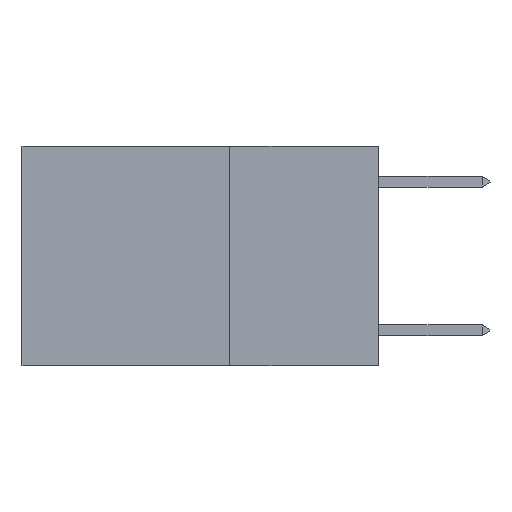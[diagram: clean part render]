
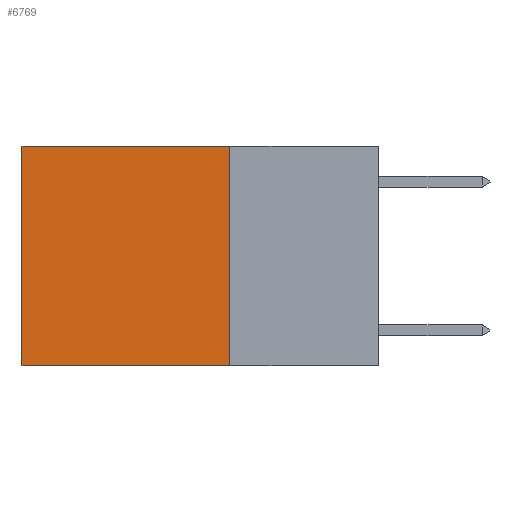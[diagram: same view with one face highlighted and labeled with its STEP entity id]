
A CAD part, left-side view. The second image highlights one B-rep face of the part: STEP entity #6769.
In plain terms, the highlighted planar face has unit normal (-1, 0, 0).
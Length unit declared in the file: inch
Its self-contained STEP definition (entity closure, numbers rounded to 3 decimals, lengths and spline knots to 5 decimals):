
#314 = CARTESIAN_POINT ( 'NONE',  ( 0.2625, 0.6, 0. ) ) ;
#1008 = DIRECTION ( 'NONE',  ( 1., 0., 0. ) ) ;
#1084 = LINE ( 'NONE', #8277, #3720 ) ;
#1279 = VERTEX_POINT ( 'NONE', #1450 ) ;
#1300 = ORIENTED_EDGE ( 'NONE', *, *, #3830, .T. ) ;
#1450 = CARTESIAN_POINT ( 'NONE',  ( 0.2625, 0.6, -0.37 ) ) ;
#1474 = DIRECTION ( 'NONE',  ( 0., 0., -1. ) ) ;
#1556 = ORIENTED_EDGE ( 'NONE', *, *, #11537, .T. ) ;
#2070 = ORIENTED_EDGE ( 'NONE', *, *, #11967, .F. ) ;
#2191 = VERTEX_POINT ( 'NONE', #4610 ) ;
#2235 = ORIENTED_EDGE ( 'NONE', *, *, #9060, .F. ) ;
#2971 = VECTOR ( 'NONE', #10011, 39.37008 ) ;
#3187 = EDGE_LOOP ( 'NONE', ( #1300, #2235, #2070, #1556 ) ) ;
#3720 = VECTOR ( 'NONE', #1474, 39.37008 ) ;
#3830 = EDGE_CURVE ( 'NONE', #10995, #1279, #5900, .T. ) ;
#4610 = CARTESIAN_POINT ( 'NONE',  ( 0.2625, 0.25, 0. ) ) ;
#4709 = DIRECTION ( 'NONE',  ( 0., 1., 0. ) ) ;
#4841 = CARTESIAN_POINT ( 'NONE',  ( 0.2625, 0.6, 0. ) ) ;
#4968 = PLANE ( 'NONE',  #10138 ) ;
#5558 = DIRECTION ( 'NONE',  ( 0., 1., 0. ) ) ;
#5900 = LINE ( 'NONE', #314, #2971 ) ;
#6769 = ADVANCED_FACE ( 'NONE', ( #7338 ), #4968, .F. ) ;
#7338 = FACE_OUTER_BOUND ( 'NONE', #3187, .T. ) ;
#7838 = DIRECTION ( 'NONE',  ( 0., 0., -1. ) ) ;
#8277 = CARTESIAN_POINT ( 'NONE',  ( 0.2625, 0.25, 0. ) ) ;
#8889 = VECTOR ( 'NONE', #4709, 39.37008 ) ;
#9060 = EDGE_CURVE ( 'NONE', #10193, #1279, #9171, .T. ) ;
#9171 = LINE ( 'NONE', #10351, #8889 ) ;
#10011 = DIRECTION ( 'NONE',  ( 0., 0., -1. ) ) ;
#10138 = AXIS2_PLACEMENT_3D ( 'NONE', #11495, #1008, #7838 ) ;
#10193 = VERTEX_POINT ( 'NONE', #11016 ) ;
#10351 = CARTESIAN_POINT ( 'NONE',  ( 0.2625, 0.25, -0.37 ) ) ;
#10995 = VERTEX_POINT ( 'NONE', #4841 ) ;
#11016 = CARTESIAN_POINT ( 'NONE',  ( 0.2625, 0.25, -0.37 ) ) ;
#11495 = CARTESIAN_POINT ( 'NONE',  ( 0.2625, 0.25, 0. ) ) ;
#11537 = EDGE_CURVE ( 'NONE', #2191, #10995, #11828, .T. ) ;
#11542 = VECTOR ( 'NONE', #5558, 39.37008 ) ;
#11828 = LINE ( 'NONE', #12053, #11542 ) ;
#11967 = EDGE_CURVE ( 'NONE', #2191, #10193, #1084, .T. ) ;
#12053 = CARTESIAN_POINT ( 'NONE',  ( 0.2625, 0.25, 0. ) ) ;
